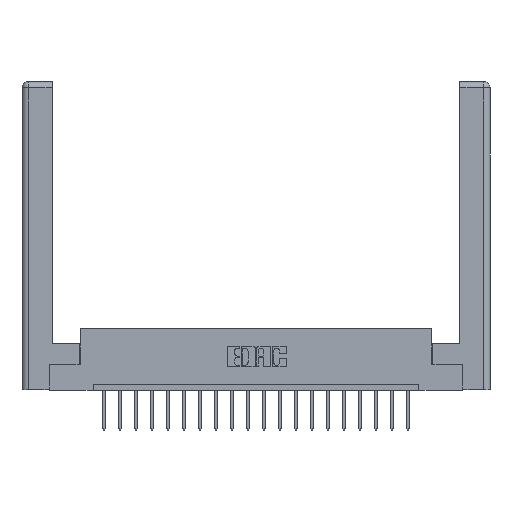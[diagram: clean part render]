
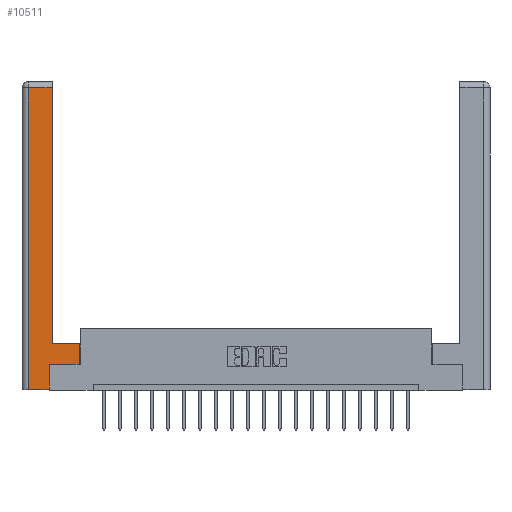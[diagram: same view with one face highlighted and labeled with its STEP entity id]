
A CAD part, top view. The second image highlights one B-rep face of the part: STEP entity #10511.
In plain terms, the highlighted planar face has unit normal (0, 0, 1).
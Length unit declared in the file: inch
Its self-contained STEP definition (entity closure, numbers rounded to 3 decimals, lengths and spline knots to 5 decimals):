
#88 = CARTESIAN_POINT ( 'NONE',  ( 0.265, 0.245, 0. ) ) ;
#120 = CARTESIAN_POINT ( 'NONE',  ( 0.295, 3., 0. ) ) ;
#209 = CARTESIAN_POINT ( 'NONE',  ( 0.0615, 0., 0. ) ) ;
#285 = VERTEX_POINT ( 'NONE', #19649 ) ;
#621 = FACE_OUTER_BOUND ( 'NONE', #15731, .T. ) ;
#676 = EDGE_CURVE ( 'NONE', #8656, #285, #5220, .T. ) ;
#902 = ORIENTED_EDGE ( 'NONE', *, *, #17212, .T. ) ;
#1136 = VECTOR ( 'NONE', #9129, 39.37008 ) ;
#1410 = VERTEX_POINT ( 'NONE', #9542 ) ;
#1780 = DIRECTION ( 'NONE',  ( 0., 1., 0. ) ) ;
#2377 = LINE ( 'NONE', #7548, #1136 ) ;
#2643 = VECTOR ( 'NONE', #8025, 39.37008 ) ;
#3173 = VERTEX_POINT ( 'NONE', #209 ) ;
#4203 = ORIENTED_EDGE ( 'NONE', *, *, #15531, .T. ) ;
#4220 = CARTESIAN_POINT ( 'NONE',  ( 0.565, 0.45, 0. ) ) ;
#4648 = DIRECTION ( 'NONE',  ( -1., 0., 0. ) ) ;
#4741 = VERTEX_POINT ( 'NONE', #14473 ) ;
#4767 = DIRECTION ( 'NONE',  ( 1., 0., 0. ) ) ;
#4819 = DIRECTION ( 'NONE',  ( 0., 0., -1. ) ) ;
#5220 = LINE ( 'NONE', #120, #9389 ) ;
#5265 = LINE ( 'NONE', #12029, #17765 ) ;
#5358 = VERTEX_POINT ( 'NONE', #4220 ) ;
#5371 = VERTEX_POINT ( 'NONE', #10831 ) ;
#5871 = CARTESIAN_POINT ( 'NONE',  ( 0.295, 0.45, 0. ) ) ;
#6063 = ORIENTED_EDGE ( 'NONE', *, *, #19743, .T. ) ;
#6551 = VECTOR ( 'NONE', #17431, 39.37008 ) ;
#6863 = LINE ( 'NONE', #18511, #18617 ) ;
#7548 = CARTESIAN_POINT ( 'NONE',  ( 0.565, 0.245, 0. ) ) ;
#7575 = VECTOR ( 'NONE', #1780, 39.37008 ) ;
#8025 = DIRECTION ( 'NONE',  ( 0., 1., 0. ) ) ;
#8028 = ORIENTED_EDGE ( 'NONE', *, *, #11677, .T. ) ;
#8240 = ORIENTED_EDGE ( 'NONE', *, *, #8904, .T. ) ;
#8656 = VERTEX_POINT ( 'NONE', #5871 ) ;
#8904 = EDGE_CURVE ( 'NONE', #5371, #5358, #12262, .T. ) ;
#9129 = DIRECTION ( 'NONE',  ( 1., 0., 0. ) ) ;
#9389 = VECTOR ( 'NONE', #15784, 39.37008 ) ;
#9542 = CARTESIAN_POINT ( 'NONE',  ( 0.265, 0., 0. ) ) ;
#9593 = DIRECTION ( 'NONE',  ( -1., 0., 0. ) ) ;
#9975 = LINE ( 'NONE', #12427, #17803 ) ;
#10186 = VERTEX_POINT ( 'NONE', #14092 ) ;
#10456 = LINE ( 'NONE', #11063, #6551 ) ;
#10511 = ADVANCED_FACE ( 'NONE', ( #621 ), #15857, .F. ) ;
#10685 = ORIENTED_EDGE ( 'NONE', *, *, #12448, .T. ) ;
#10831 = CARTESIAN_POINT ( 'NONE',  ( 0.565, 0.245, 0. ) ) ;
#11063 = CARTESIAN_POINT ( 'NONE',  ( 0.295, 0.45, 0. ) ) ;
#11677 = EDGE_CURVE ( 'NONE', #3173, #1410, #9975, .T. ) ;
#11826 = DIRECTION ( 'NONE',  ( 0., -1., 0. ) ) ;
#12029 = CARTESIAN_POINT ( 'NONE',  ( 0.0615, 0., 0. ) ) ;
#12262 = LINE ( 'NONE', #15999, #7575 ) ;
#12427 = CARTESIAN_POINT ( 'NONE',  ( 0.265, 0., 0. ) ) ;
#12448 = EDGE_CURVE ( 'NONE', #4741, #3173, #5265, .T. ) ;
#12599 = ORIENTED_EDGE ( 'NONE', *, *, #15610, .T. ) ;
#14092 = CARTESIAN_POINT ( 'NONE',  ( 0.265, 0.245, 0. ) ) ;
#14278 = CARTESIAN_POINT ( 'NONE',  ( 0., 0., 0. ) ) ;
#14473 = CARTESIAN_POINT ( 'NONE',  ( 0.0615, 2.94, 0. ) ) ;
#15531 = EDGE_CURVE ( 'NONE', #285, #4741, #6863, .T. ) ;
#15610 = EDGE_CURVE ( 'NONE', #1410, #10186, #18134, .T. ) ;
#15731 = EDGE_LOOP ( 'NONE', ( #20153, #4203, #10685, #8028, #12599, #6063, #8240, #902 ) ) ;
#15784 = DIRECTION ( 'NONE',  ( 0., 1., 0. ) ) ;
#15844 = AXIS2_PLACEMENT_3D ( 'NONE', #14278, #4819, #9593 ) ;
#15857 = PLANE ( 'NONE',  #15844 ) ;
#15999 = CARTESIAN_POINT ( 'NONE',  ( 0.565, 0.45, 0. ) ) ;
#17212 = EDGE_CURVE ( 'NONE', #5358, #8656, #10456, .T. ) ;
#17431 = DIRECTION ( 'NONE',  ( -1., 0., 0. ) ) ;
#17765 = VECTOR ( 'NONE', #11826, 39.37008 ) ;
#17803 = VECTOR ( 'NONE', #4767, 39.37008 ) ;
#18134 = LINE ( 'NONE', #88, #2643 ) ;
#18511 = CARTESIAN_POINT ( 'NONE',  ( 0.0615, 2.94, 0. ) ) ;
#18617 = VECTOR ( 'NONE', #4648, 39.37008 ) ;
#19649 = CARTESIAN_POINT ( 'NONE',  ( 0.295, 2.94, 0. ) ) ;
#19743 = EDGE_CURVE ( 'NONE', #10186, #5371, #2377, .T. ) ;
#20153 = ORIENTED_EDGE ( 'NONE', *, *, #676, .T. ) ;
